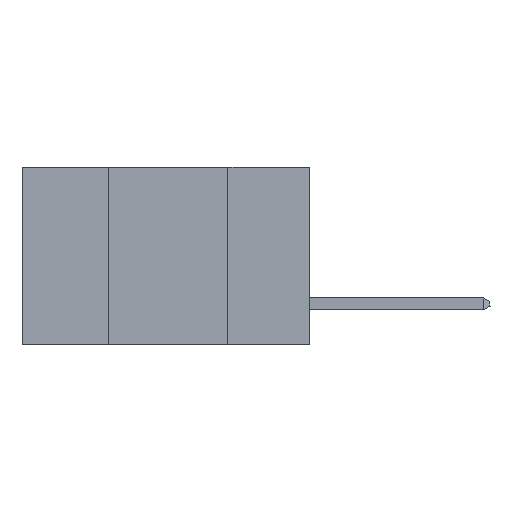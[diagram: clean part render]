
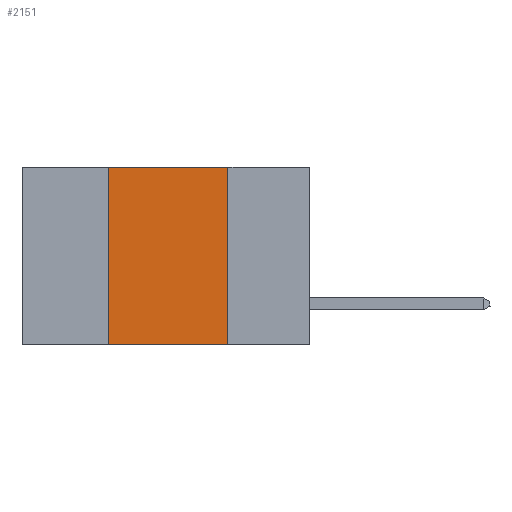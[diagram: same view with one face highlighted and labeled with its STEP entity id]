
A CAD part, left-side view. The second image highlights one B-rep face of the part: STEP entity #2151.
In plain terms, the highlighted planar face has unit normal (-1, 0, 0).
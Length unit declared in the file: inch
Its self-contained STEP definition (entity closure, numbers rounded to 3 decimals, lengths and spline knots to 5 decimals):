
#1715 = VERTEX_POINT ( 'NONE', #7569 ) ;
#1836 = LINE ( 'NONE', #14818, #2466 ) ;
#2021 = VECTOR ( 'NONE', #8562, 39.37008 ) ;
#2060 = VERTEX_POINT ( 'NONE', #21579 ) ;
#2151 = ADVANCED_FACE ( 'NONE', ( #4743 ), #7546, .F. ) ;
#2466 = VECTOR ( 'NONE', #8475, 39.37008 ) ;
#2574 = EDGE_LOOP ( 'NONE', ( #6556, #24102, #10568, #15974 ) ) ;
#2613 = CARTESIAN_POINT ( 'NONE',  ( 0., 0.17, -0.37 ) ) ;
#2872 = VERTEX_POINT ( 'NONE', #6580 ) ;
#2956 = VERTEX_POINT ( 'NONE', #2613 ) ;
#4280 = AXIS2_PLACEMENT_3D ( 'NONE', #5749, #18231, #5651 ) ;
#4689 = CARTESIAN_POINT ( 'NONE',  ( 0., 0.6, 0. ) ) ;
#4743 = FACE_OUTER_BOUND ( 'NONE', #2574, .T. ) ;
#5651 = DIRECTION ( 'NONE',  ( 0., 0., -1. ) ) ;
#5749 = CARTESIAN_POINT ( 'NONE',  ( 0., 0.6, 0. ) ) ;
#5789 = EDGE_CURVE ( 'NONE', #1715, #2956, #1836, .T. ) ;
#6556 = ORIENTED_EDGE ( 'NONE', *, *, #5789, .F. ) ;
#6580 = CARTESIAN_POINT ( 'NONE',  ( 0., 0.42, -0.37 ) ) ;
#7546 = PLANE ( 'NONE',  #4280 ) ;
#7569 = CARTESIAN_POINT ( 'NONE',  ( 0., 0.17, 0. ) ) ;
#8083 = EDGE_CURVE ( 'NONE', #2060, #1715, #25306, .T. ) ;
#8475 = DIRECTION ( 'NONE',  ( 0., 0., -1. ) ) ;
#8562 = DIRECTION ( 'NONE',  ( 0., -1., 0. ) ) ;
#9613 = CARTESIAN_POINT ( 'NONE',  ( 0., 0.6, -0.37 ) ) ;
#10313 = VECTOR ( 'NONE', #20677, 39.37008 ) ;
#10568 = ORIENTED_EDGE ( 'NONE', *, *, #19279, .F. ) ;
#11649 = LINE ( 'NONE', #21041, #10313 ) ;
#13703 = DIRECTION ( 'NONE',  ( 0., -1., 0. ) ) ;
#14818 = CARTESIAN_POINT ( 'NONE',  ( 0., 0.17, 0. ) ) ;
#15974 = ORIENTED_EDGE ( 'NONE', *, *, #18197, .T. ) ;
#16862 = LINE ( 'NONE', #9613, #21401 ) ;
#18197 = EDGE_CURVE ( 'NONE', #2872, #2956, #16862, .T. ) ;
#18231 = DIRECTION ( 'NONE',  ( 1., 0., 0. ) ) ;
#19279 = EDGE_CURVE ( 'NONE', #2872, #2060, #11649, .T. ) ;
#20677 = DIRECTION ( 'NONE',  ( 0., 0., 1. ) ) ;
#21041 = CARTESIAN_POINT ( 'NONE',  ( 0., 0.42, 0. ) ) ;
#21401 = VECTOR ( 'NONE', #13703, 39.37008 ) ;
#21579 = CARTESIAN_POINT ( 'NONE',  ( 0., 0.42, 0. ) ) ;
#24102 = ORIENTED_EDGE ( 'NONE', *, *, #8083, .F. ) ;
#25306 = LINE ( 'NONE', #4689, #2021 ) ;
